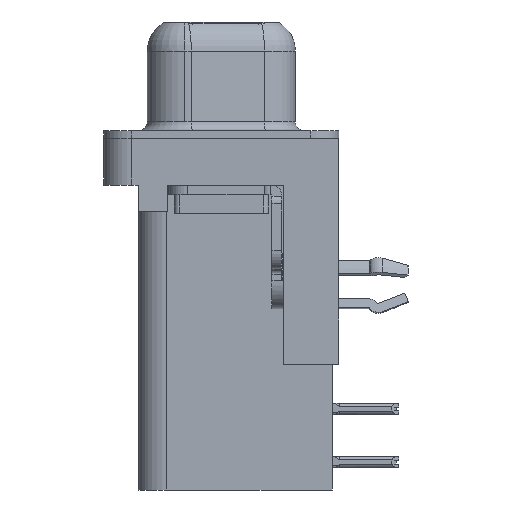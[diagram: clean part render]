
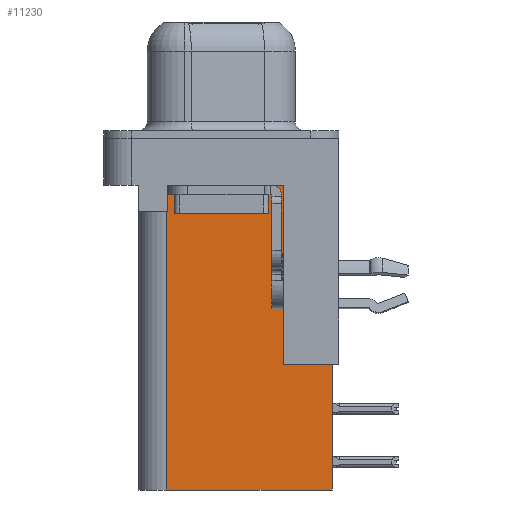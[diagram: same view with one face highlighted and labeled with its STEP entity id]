
A CAD part, left-side view. The second image highlights one B-rep face of the part: STEP entity #11230.
In plain terms, the highlighted planar face has unit normal (-1, 0, 0).
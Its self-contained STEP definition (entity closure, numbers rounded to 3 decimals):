
#734 = CARTESIAN_POINT ( 'NONE',  ( 3.79, -5.925, -2. ) ) ;
#957 = VERTEX_POINT ( 'NONE', #3132 ) ;
#974 = LINE ( 'NONE', #12604, #996 ) ;
#996 = VECTOR ( 'NONE', #6656, 1000. ) ;
#2142 = DIRECTION ( 'NONE',  ( 0., 1., 0. ) ) ;
#2883 = AXIS2_PLACEMENT_3D ( 'NONE', #9841, #13922, #2142 ) ;
#3045 = CARTESIAN_POINT ( 'NONE',  ( 3.79, -3.295, -18.76 ) ) ;
#3132 = CARTESIAN_POINT ( 'NONE',  ( 3.79, -5.925, -12.05 ) ) ;
#3194 = VERTEX_POINT ( 'NONE', #10228 ) ;
#3603 = EDGE_CURVE ( 'NONE', #20338, #12078, #16918, .T. ) ;
#5667 = CARTESIAN_POINT ( 'NONE',  ( 3.79, -3.295, -18.76 ) ) ;
#5797 = CARTESIAN_POINT ( 'NONE',  ( 3.79, 0., -3.9 ) ) ;
#5801 = ORIENTED_EDGE ( 'NONE', *, *, #21358, .T. ) ;
#6199 = CARTESIAN_POINT ( 'NONE',  ( 3.79, -6.295, -12.05 ) ) ;
#6287 = DIRECTION ( 'NONE',  ( 0., 1., 0. ) ) ;
#6656 = DIRECTION ( 'NONE',  ( 0., 1., 0. ) ) ;
#6798 = ORIENTED_EDGE ( 'NONE', *, *, #3603, .F. ) ;
#7174 = ORIENTED_EDGE ( 'NONE', *, *, #9658, .F. ) ;
#8621 = VERTEX_POINT ( 'NONE', #23851 ) ;
#8694 = DIRECTION ( 'NONE',  ( 0., 0., 1. ) ) ;
#9363 = EDGE_CURVE ( 'NONE', #10819, #20578, #20948, .T. ) ;
#9658 = EDGE_CURVE ( 'NONE', #12078, #20578, #19845, .T. ) ;
#9841 = CARTESIAN_POINT ( 'NONE',  ( 3.79, -3.295, -18.76 ) ) ;
#10228 = CARTESIAN_POINT ( 'NONE',  ( 3.79, -3.295, -12.05 ) ) ;
#10396 = VECTOR ( 'NONE', #8694, 1000. ) ;
#10443 = VECTOR ( 'NONE', #20462, 1000. ) ;
#10447 = LINE ( 'NONE', #3045, #10396 ) ;
#10564 = LINE ( 'NONE', #734, #10443 ) ;
#10819 = VERTEX_POINT ( 'NONE', #16310 ) ;
#10932 = ORIENTED_EDGE ( 'NONE', *, *, #24019, .F. ) ;
#11230 = ADVANCED_FACE ( 'NONE', ( #13963 ), #15872, .F. ) ;
#12078 = VERTEX_POINT ( 'NONE', #19300 ) ;
#12604 = CARTESIAN_POINT ( 'NONE',  ( 3.79, -3.295, -2.5 ) ) ;
#13446 = EDGE_LOOP ( 'NONE', ( #21014, #22611, #19191, #7174, #6798, #10932, #5801, #16166 ) ) ;
#13507 = VECTOR ( 'NONE', #19137, 1000. ) ;
#13866 = LINE ( 'NONE', #21160, #13507 ) ;
#13922 = DIRECTION ( 'NONE',  ( 1., 0., 0. ) ) ;
#13963 = FACE_OUTER_BOUND ( 'NONE', #13446, .T. ) ;
#14273 = CARTESIAN_POINT ( 'NONE',  ( 3.79, 2.925, -18.76 ) ) ;
#14819 = CARTESIAN_POINT ( 'NONE',  ( 3.79, -5.925, -18.76 ) ) ;
#15049 = EDGE_CURVE ( 'NONE', #24855, #8621, #974, .T. ) ;
#15872 = PLANE ( 'NONE',  #2883 ) ;
#16166 = ORIENTED_EDGE ( 'NONE', *, *, #17324, .T. ) ;
#16310 = CARTESIAN_POINT ( 'NONE',  ( 3.79, 2.895, -3.9 ) ) ;
#16824 = VECTOR ( 'NONE', #21573, 1000. ) ;
#16852 = EDGE_CURVE ( 'NONE', #8621, #10819, #13866, .T. ) ;
#16918 = LINE ( 'NONE', #5667, #16824 ) ;
#17324 = EDGE_CURVE ( 'NONE', #3194, #24855, #10447, .T. ) ;
#17671 = DIRECTION ( 'NONE',  ( 0., 1., 0. ) ) ;
#17919 = CARTESIAN_POINT ( 'NONE',  ( 3.79, -3.295, -2.5 ) ) ;
#18033 = VECTOR ( 'NONE', #6287, 1000. ) ;
#18086 = LINE ( 'NONE', #6199, #18033 ) ;
#19137 = DIRECTION ( 'NONE',  ( 0., 0., -1. ) ) ;
#19191 = ORIENTED_EDGE ( 'NONE', *, *, #9363, .T. ) ;
#19300 = CARTESIAN_POINT ( 'NONE',  ( 3.79, 2.925, -18.76 ) ) ;
#19699 = VECTOR ( 'NONE', #20304, 1000. ) ;
#19845 = LINE ( 'NONE', #14273, #19699 ) ;
#20304 = DIRECTION ( 'NONE',  ( 0., 0., 1. ) ) ;
#20338 = VERTEX_POINT ( 'NONE', #14819 ) ;
#20462 = DIRECTION ( 'NONE',  ( 0., 0., -1. ) ) ;
#20578 = VERTEX_POINT ( 'NONE', #23351 ) ;
#20779 = VECTOR ( 'NONE', #17671, 1000. ) ;
#20948 = LINE ( 'NONE', #5797, #20779 ) ;
#21014 = ORIENTED_EDGE ( 'NONE', *, *, #15049, .T. ) ;
#21160 = CARTESIAN_POINT ( 'NONE',  ( 3.79, 2.895, -3.9 ) ) ;
#21358 = EDGE_CURVE ( 'NONE', #957, #3194, #18086, .T. ) ;
#21573 = DIRECTION ( 'NONE',  ( 0., 1., 0. ) ) ;
#22611 = ORIENTED_EDGE ( 'NONE', *, *, #16852, .T. ) ;
#23351 = CARTESIAN_POINT ( 'NONE',  ( 3.79, 2.925, -3.9 ) ) ;
#23851 = CARTESIAN_POINT ( 'NONE',  ( 3.79, 2.895, -2.5 ) ) ;
#24019 = EDGE_CURVE ( 'NONE', #957, #20338, #10564, .T. ) ;
#24855 = VERTEX_POINT ( 'NONE', #17919 ) ;
